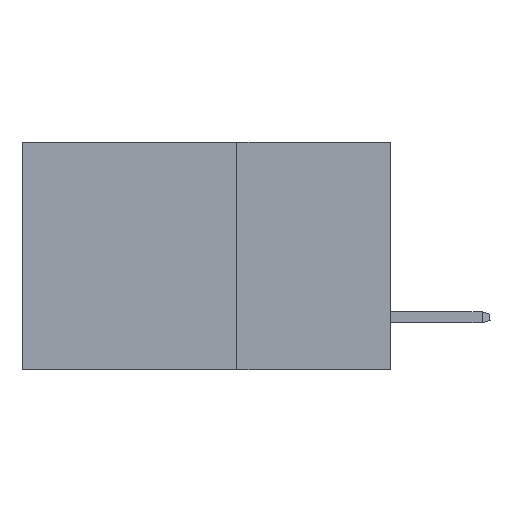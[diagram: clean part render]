
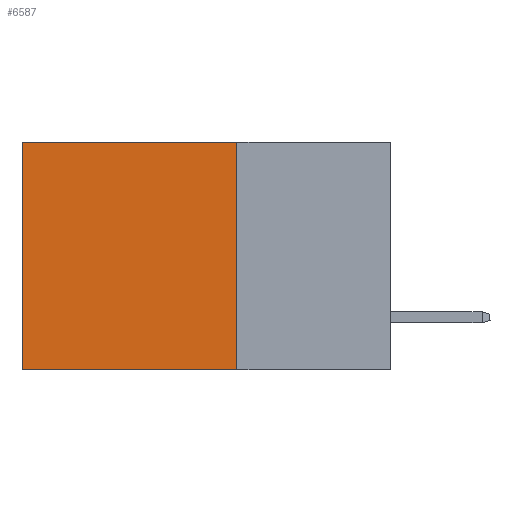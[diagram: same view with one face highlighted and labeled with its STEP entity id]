
A CAD part, left-side view. The second image highlights one B-rep face of the part: STEP entity #6587.
In plain terms, the highlighted planar face has unit normal (-1, 0, 0).
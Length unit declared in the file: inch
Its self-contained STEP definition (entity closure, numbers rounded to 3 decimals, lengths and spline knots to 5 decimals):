
#444 = CARTESIAN_POINT ( 'NONE',  ( 0.2875, 0.25, -0.37 ) ) ;
#5000 = PLANE ( 'NONE',  #5189 ) ;
#5189 = AXIS2_PLACEMENT_3D ( 'NONE', #38357, #14709, #22802 ) ;
#6587 = ADVANCED_FACE ( 'NONE', ( #17275 ), #5000, .F. ) ;
#8437 = VECTOR ( 'NONE', #33732, 39.37008 ) ;
#10640 = DIRECTION ( 'NONE',  ( 0., 1., 0. ) ) ;
#11144 = CARTESIAN_POINT ( 'NONE',  ( 0.2875, 0.6, 0. ) ) ;
#11857 = LINE ( 'NONE', #19503, #26263 ) ;
#12580 = EDGE_LOOP ( 'NONE', ( #34753, #20155, #41363, #33690 ) ) ;
#14709 = DIRECTION ( 'NONE',  ( 1., 0., 0. ) ) ;
#17137 = DIRECTION ( 'NONE',  ( 0., 0., -1. ) ) ;
#17275 = FACE_OUTER_BOUND ( 'NONE', #12580, .T. ) ;
#18362 = VERTEX_POINT ( 'NONE', #444 ) ;
#19488 = VECTOR ( 'NONE', #10640, 39.37008 ) ;
#19503 = CARTESIAN_POINT ( 'NONE',  ( 0.2875, 0.25, 0. ) ) ;
#19741 = LINE ( 'NONE', #30561, #8437 ) ;
#20155 = ORIENTED_EDGE ( 'NONE', *, *, #27949, .F. ) ;
#20489 = VERTEX_POINT ( 'NONE', #27713 ) ;
#22197 = CARTESIAN_POINT ( 'NONE',  ( 0.2875, 0.6, 0. ) ) ;
#22802 = DIRECTION ( 'NONE',  ( 0., 0., -1. ) ) ;
#24086 = VERTEX_POINT ( 'NONE', #22197 ) ;
#25238 = EDGE_CURVE ( 'NONE', #33193, #24086, #36053, .T. ) ;
#25863 = VECTOR ( 'NONE', #40620, 39.37008 ) ;
#26263 = VECTOR ( 'NONE', #17137, 39.37008 ) ;
#27713 = CARTESIAN_POINT ( 'NONE',  ( 0.2875, 0.6, -0.37 ) ) ;
#27949 = EDGE_CURVE ( 'NONE', #18362, #20489, #19741, .T. ) ;
#30257 = CARTESIAN_POINT ( 'NONE',  ( 0.2875, 0.25, 0. ) ) ;
#30561 = CARTESIAN_POINT ( 'NONE',  ( 0.2875, 0.25, -0.37 ) ) ;
#32008 = EDGE_CURVE ( 'NONE', #24086, #20489, #34642, .T. ) ;
#33193 = VERTEX_POINT ( 'NONE', #35444 ) ;
#33690 = ORIENTED_EDGE ( 'NONE', *, *, #25238, .T. ) ;
#33732 = DIRECTION ( 'NONE',  ( 0., 1., 0. ) ) ;
#34642 = LINE ( 'NONE', #11144, #25863 ) ;
#34753 = ORIENTED_EDGE ( 'NONE', *, *, #32008, .T. ) ;
#35444 = CARTESIAN_POINT ( 'NONE',  ( 0.2875, 0.25, 0. ) ) ;
#36053 = LINE ( 'NONE', #30257, #19488 ) ;
#36802 = EDGE_CURVE ( 'NONE', #33193, #18362, #11857, .T. ) ;
#38357 = CARTESIAN_POINT ( 'NONE',  ( 0.2875, 0.25, 0. ) ) ;
#40620 = DIRECTION ( 'NONE',  ( 0., 0., -1. ) ) ;
#41363 = ORIENTED_EDGE ( 'NONE', *, *, #36802, .F. ) ;
